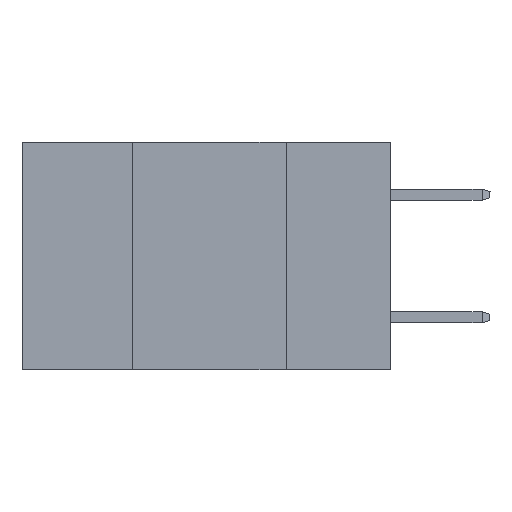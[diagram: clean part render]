
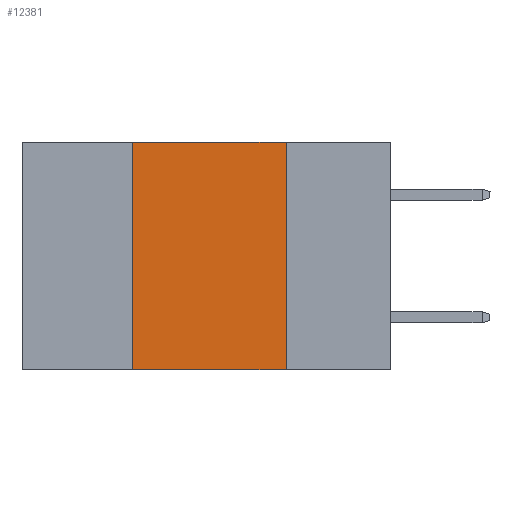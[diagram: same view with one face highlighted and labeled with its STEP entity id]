
A CAD part, left-side view. The second image highlights one B-rep face of the part: STEP entity #12381.
In plain terms, the highlighted planar face has unit normal (-1, 0, 0).
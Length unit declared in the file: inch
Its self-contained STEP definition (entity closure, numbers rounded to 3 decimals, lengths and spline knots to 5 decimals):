
#866 = EDGE_CURVE ( 'NONE', #3083, #3411, #18338, .T. ) ;
#2530 = DIRECTION ( 'NONE',  ( 0., -1., 0. ) ) ;
#2574 = EDGE_CURVE ( 'NONE', #2835, #15515, #11800, .T. ) ;
#2814 = CARTESIAN_POINT ( 'NONE',  ( 0., 0.42, 0. ) ) ;
#2835 = VERTEX_POINT ( 'NONE', #17683 ) ;
#3083 = VERTEX_POINT ( 'NONE', #20864 ) ;
#3269 = DIRECTION ( 'NONE',  ( 0., -1., 0. ) ) ;
#3313 = CARTESIAN_POINT ( 'NONE',  ( 0., 0.42, 0. ) ) ;
#3411 = VERTEX_POINT ( 'NONE', #3313 ) ;
#3656 = EDGE_CURVE ( 'NONE', #3083, #15515, #16267, .T. ) ;
#4816 = ORIENTED_EDGE ( 'NONE', *, *, #18308, .F. ) ;
#4948 = DIRECTION ( 'NONE',  ( 0., 0., -1. ) ) ;
#5534 = VECTOR ( 'NONE', #4948, 39.37008 ) ;
#6029 = DIRECTION ( 'NONE',  ( 0., 0., 1. ) ) ;
#6609 = CARTESIAN_POINT ( 'NONE',  ( 0., 0.17, 0. ) ) ;
#6713 = ORIENTED_EDGE ( 'NONE', *, *, #3656, .T. ) ;
#7558 = FACE_OUTER_BOUND ( 'NONE', #19887, .T. ) ;
#10442 = DIRECTION ( 'NONE',  ( 1., 0., 0. ) ) ;
#10934 = AXIS2_PLACEMENT_3D ( 'NONE', #18889, #10442, #17223 ) ;
#11765 = VECTOR ( 'NONE', #3269, 39.37008 ) ;
#11800 = LINE ( 'NONE', #6609, #5534 ) ;
#12381 = ADVANCED_FACE ( 'NONE', ( #7558 ), #20559, .F. ) ;
#13678 = ORIENTED_EDGE ( 'NONE', *, *, #866, .F. ) ;
#15008 = CARTESIAN_POINT ( 'NONE',  ( 0., 0.6, 0. ) ) ;
#15515 = VERTEX_POINT ( 'NONE', #20537 ) ;
#16267 = LINE ( 'NONE', #17711, #17996 ) ;
#17223 = DIRECTION ( 'NONE',  ( 0., 0., -1. ) ) ;
#17683 = CARTESIAN_POINT ( 'NONE',  ( 0., 0.17, 0. ) ) ;
#17711 = CARTESIAN_POINT ( 'NONE',  ( 0., 0.6, -0.37 ) ) ;
#17996 = VECTOR ( 'NONE', #2530, 39.37008 ) ;
#18308 = EDGE_CURVE ( 'NONE', #3411, #2835, #20572, .T. ) ;
#18338 = LINE ( 'NONE', #2814, #18726 ) ;
#18694 = ORIENTED_EDGE ( 'NONE', *, *, #2574, .F. ) ;
#18726 = VECTOR ( 'NONE', #6029, 39.37008 ) ;
#18889 = CARTESIAN_POINT ( 'NONE',  ( 0., 0.6, 0. ) ) ;
#19887 = EDGE_LOOP ( 'NONE', ( #18694, #4816, #13678, #6713 ) ) ;
#20537 = CARTESIAN_POINT ( 'NONE',  ( 0., 0.17, -0.37 ) ) ;
#20559 = PLANE ( 'NONE',  #10934 ) ;
#20572 = LINE ( 'NONE', #15008, #11765 ) ;
#20864 = CARTESIAN_POINT ( 'NONE',  ( 0., 0.42, -0.37 ) ) ;
